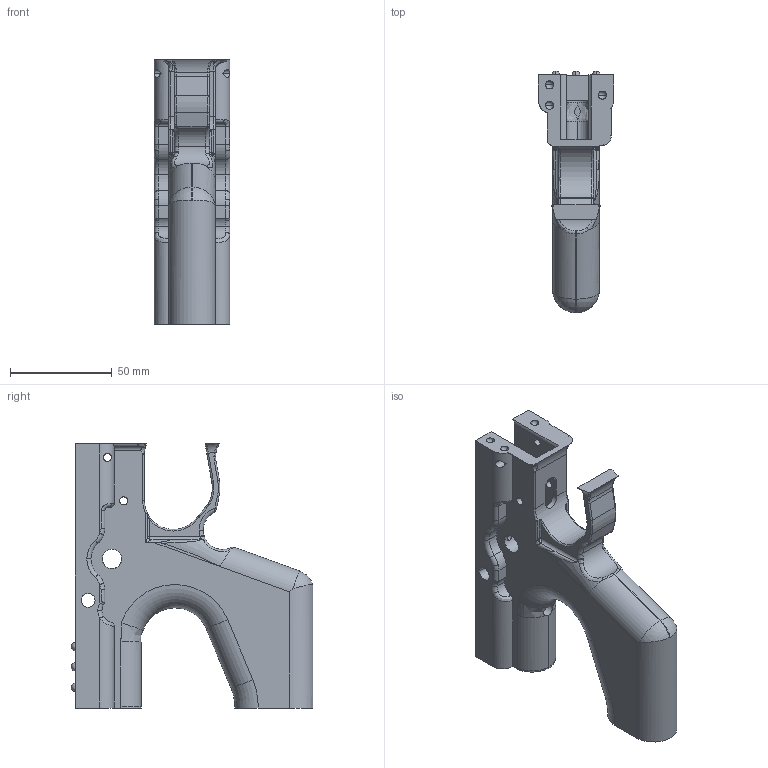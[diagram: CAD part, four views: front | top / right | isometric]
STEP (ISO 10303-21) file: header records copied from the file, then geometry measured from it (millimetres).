
FILE_DESCRIPTION (( 'STEP AP214' ), '1' );
FILE_NAME ('Grip_2_1.step', '2019-12-18T03:07:48', ( '' ), ( '' ), 'SwSTEP 2.0', 'SolidWorks 2019', '' );
FILE_SCHEMA (( 'AUTOMOTIVE_DESIGN' ));
Length unit declared in the file: millimetre
Products named in the file (1): Grip_2_1
Bounding box: 37.13 x 119.02 x 130 mm (x, y, z)
Volume: 190783.4 mm3; surface area: 40645.6 mm2
Topology: 1 solids, 1 shells, 307 faces, 883 edges, 541 vertices
Faces by surface type: cylinder 111, bspline 59, sphere 50, torus 47, plane 40
Entity records: 14199 total; most frequent: CARTESIAN_POINT 7023, ORIENTED_EDGE 1564, DIRECTION 1447, EDGE_CURVE 782, AXIS2_PLACEMENT_3D 614, VERTEX_POINT 495, CIRCLE 365, EDGE_LOOP 347
